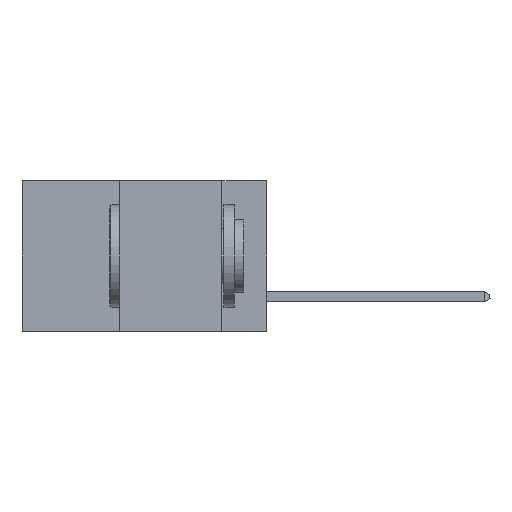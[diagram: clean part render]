
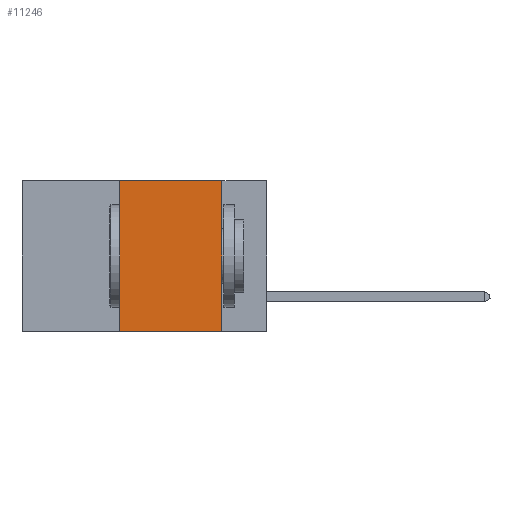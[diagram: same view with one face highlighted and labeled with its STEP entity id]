
A CAD part, left-side view. The second image highlights one B-rep face of the part: STEP entity #11246.
In plain terms, the highlighted planar face has unit normal (-1, 0, 0).
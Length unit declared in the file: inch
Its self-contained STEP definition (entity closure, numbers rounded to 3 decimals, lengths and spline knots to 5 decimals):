
#1524 = CARTESIAN_POINT ( 'NONE',  ( 0., 0.11, 0. ) ) ;
#2703 = VECTOR ( 'NONE', #5259, 39.37008 ) ;
#2949 = DIRECTION ( 'NONE',  ( 0., 0., 1. ) ) ;
#2989 = CARTESIAN_POINT ( 'NONE',  ( 0., 0.11, -0.37 ) ) ;
#3012 = VERTEX_POINT ( 'NONE', #1524 ) ;
#3103 = DIRECTION ( 'NONE',  ( 1., 0., 0. ) ) ;
#3160 = CARTESIAN_POINT ( 'NONE',  ( 0., 0.36, -0.37 ) ) ;
#3251 = DIRECTION ( 'NONE',  ( 0., 0., -1. ) ) ;
#4196 = EDGE_CURVE ( 'NONE', #7473, #7890, #7632, .T. ) ;
#4446 = EDGE_LOOP ( 'NONE', ( #6404, #10685, #10743, #5998 ) ) ;
#4546 = VECTOR ( 'NONE', #13791, 39.37008 ) ;
#4749 = LINE ( 'NONE', #6313, #7929 ) ;
#5259 = DIRECTION ( 'NONE',  ( 0., -1., 0. ) ) ;
#5750 = CARTESIAN_POINT ( 'NONE',  ( 0., 0.36, 0. ) ) ;
#5998 = ORIENTED_EDGE ( 'NONE', *, *, #4196, .T. ) ;
#6313 = CARTESIAN_POINT ( 'NONE',  ( 0., 0.36, 0. ) ) ;
#6404 = ORIENTED_EDGE ( 'NONE', *, *, #8398, .F. ) ;
#6419 = EDGE_CURVE ( 'NONE', #7337, #3012, #14039, .T. ) ;
#6633 = CARTESIAN_POINT ( 'NONE',  ( 0., 0.6, -0.37 ) ) ;
#7337 = VERTEX_POINT ( 'NONE', #5750 ) ;
#7473 = VERTEX_POINT ( 'NONE', #3160 ) ;
#7492 = FACE_OUTER_BOUND ( 'NONE', #4446, .T. ) ;
#7632 = LINE ( 'NONE', #6633, #2703 ) ;
#7890 = VERTEX_POINT ( 'NONE', #2989 ) ;
#7929 = VECTOR ( 'NONE', #2949, 39.37008 ) ;
#7931 = CARTESIAN_POINT ( 'NONE',  ( 0., 0.11, 0. ) ) ;
#8398 = EDGE_CURVE ( 'NONE', #3012, #7890, #11244, .T. ) ;
#8428 = VECTOR ( 'NONE', #13118, 39.37008 ) ;
#8701 = CARTESIAN_POINT ( 'NONE',  ( 0., 0.6, 0. ) ) ;
#9705 = CARTESIAN_POINT ( 'NONE',  ( 0., 0.6, 0. ) ) ;
#10685 = ORIENTED_EDGE ( 'NONE', *, *, #6419, .F. ) ;
#10743 = ORIENTED_EDGE ( 'NONE', *, *, #13708, .F. ) ;
#11244 = LINE ( 'NONE', #7931, #4546 ) ;
#11246 = ADVANCED_FACE ( 'NONE', ( #7492 ), #12275, .F. ) ;
#12275 = PLANE ( 'NONE',  #12646 ) ;
#12646 = AXIS2_PLACEMENT_3D ( 'NONE', #8701, #3103, #3251 ) ;
#13118 = DIRECTION ( 'NONE',  ( 0., -1., 0. ) ) ;
#13708 = EDGE_CURVE ( 'NONE', #7473, #7337, #4749, .T. ) ;
#13791 = DIRECTION ( 'NONE',  ( 0., 0., -1. ) ) ;
#14039 = LINE ( 'NONE', #9705, #8428 ) ;
